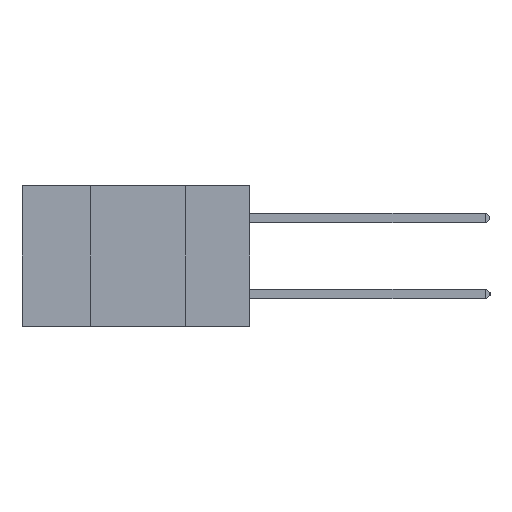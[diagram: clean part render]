
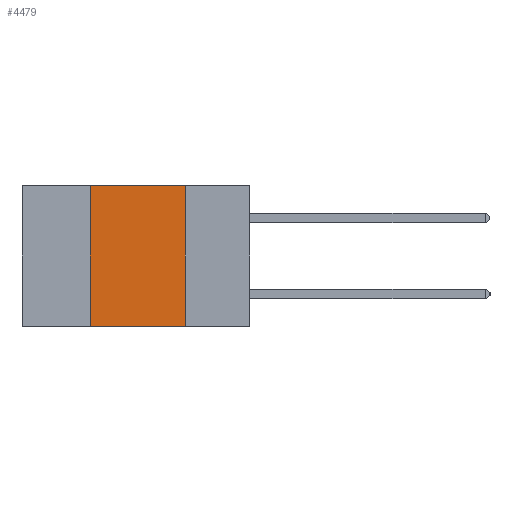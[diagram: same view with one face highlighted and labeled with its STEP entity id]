
A CAD part, left-side view. The second image highlights one B-rep face of the part: STEP entity #4479.
In plain terms, the highlighted planar face has unit normal (-1, 0, 0).
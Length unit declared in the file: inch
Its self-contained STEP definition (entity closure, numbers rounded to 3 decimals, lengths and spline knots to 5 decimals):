
#1636 = CARTESIAN_POINT ( 'NONE',  ( 0., 0.42, 0. ) ) ;
#1910 = EDGE_CURVE ( 'NONE', #20735, #13760, #7947, .T. ) ;
#2001 = LINE ( 'NONE', #5895, #14561 ) ;
#2125 = ORIENTED_EDGE ( 'NONE', *, *, #1910, .F. ) ;
#2643 = ORIENTED_EDGE ( 'NONE', *, *, #14089, .T. ) ;
#2872 = DIRECTION ( 'NONE',  ( 0., 0., -1. ) ) ;
#3190 = PLANE ( 'NONE',  #6026 ) ;
#3324 = FACE_OUTER_BOUND ( 'NONE', #19062, .T. ) ;
#3394 = DIRECTION ( 'NONE',  ( 1., 0., 0. ) ) ;
#3449 = VECTOR ( 'NONE', #4910, 39.37008 ) ;
#3542 = CARTESIAN_POINT ( 'NONE',  ( 0., 0.6, 0. ) ) ;
#4479 = ADVANCED_FACE ( 'NONE', ( #3324 ), #3190, .F. ) ;
#4910 = DIRECTION ( 'NONE',  ( 0., 0., 1. ) ) ;
#5895 = CARTESIAN_POINT ( 'NONE',  ( 0., 0.6, -0.37 ) ) ;
#6026 = AXIS2_PLACEMENT_3D ( 'NONE', #3542, #3394, #2872 ) ;
#6816 = CARTESIAN_POINT ( 'NONE',  ( 0., 0.17, 0. ) ) ;
#7947 = LINE ( 'NONE', #20819, #3449 ) ;
#10326 = LINE ( 'NONE', #21291, #14953 ) ;
#11231 = VERTEX_POINT ( 'NONE', #6816 ) ;
#11385 = VECTOR ( 'NONE', #15843, 39.37008 ) ;
#11789 = VERTEX_POINT ( 'NONE', #19821 ) ;
#12058 = EDGE_CURVE ( 'NONE', #11231, #11789, #17059, .T. ) ;
#12902 = DIRECTION ( 'NONE',  ( 0., -1., 0. ) ) ;
#13760 = VERTEX_POINT ( 'NONE', #1636 ) ;
#14089 = EDGE_CURVE ( 'NONE', #20735, #11789, #2001, .T. ) ;
#14116 = CARTESIAN_POINT ( 'NONE',  ( 0., 0.17, 0. ) ) ;
#14561 = VECTOR ( 'NONE', #17866, 39.37008 ) ;
#14953 = VECTOR ( 'NONE', #12902, 39.37008 ) ;
#15186 = CARTESIAN_POINT ( 'NONE',  ( 0., 0.42, -0.37 ) ) ;
#15243 = ORIENTED_EDGE ( 'NONE', *, *, #12058, .F. ) ;
#15843 = DIRECTION ( 'NONE',  ( 0., 0., -1. ) ) ;
#17059 = LINE ( 'NONE', #14116, #11385 ) ;
#17866 = DIRECTION ( 'NONE',  ( 0., -1., 0. ) ) ;
#19062 = EDGE_LOOP ( 'NONE', ( #15243, #19659, #2125, #2643 ) ) ;
#19659 = ORIENTED_EDGE ( 'NONE', *, *, #19791, .F. ) ;
#19791 = EDGE_CURVE ( 'NONE', #13760, #11231, #10326, .T. ) ;
#19821 = CARTESIAN_POINT ( 'NONE',  ( 0., 0.17, -0.37 ) ) ;
#20735 = VERTEX_POINT ( 'NONE', #15186 ) ;
#20819 = CARTESIAN_POINT ( 'NONE',  ( 0., 0.42, 0. ) ) ;
#21291 = CARTESIAN_POINT ( 'NONE',  ( 0., 0.6, 0. ) ) ;
